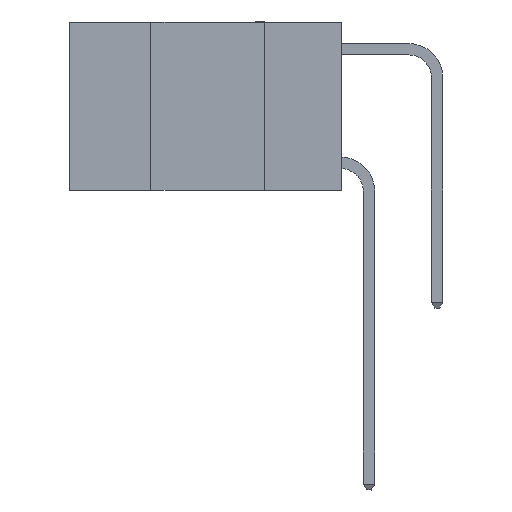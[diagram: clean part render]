
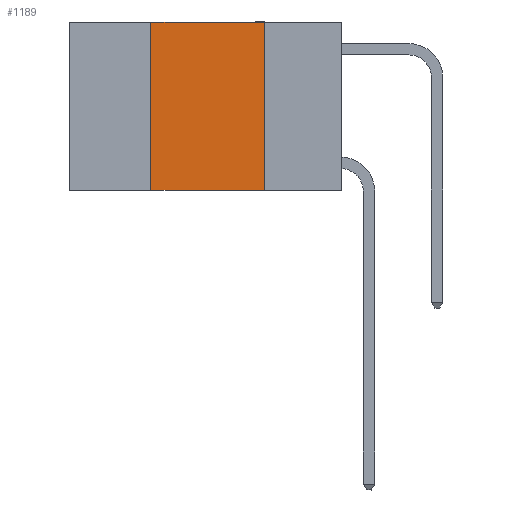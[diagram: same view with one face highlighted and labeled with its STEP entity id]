
A CAD part, left-side view. The second image highlights one B-rep face of the part: STEP entity #1189.
In plain terms, the highlighted planar face has unit normal (-1, 0, 0).
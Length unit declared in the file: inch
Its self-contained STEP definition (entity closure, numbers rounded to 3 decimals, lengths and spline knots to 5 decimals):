
#55 = EDGE_CURVE ( 'NONE', #11336, #14177, #9140, .T. ) ;
#119 = CARTESIAN_POINT ( 'NONE',  ( 0., 0.17, 0. ) ) ;
#1168 = CARTESIAN_POINT ( 'NONE',  ( 0., 0.42, -0.37 ) ) ;
#1189 = ADVANCED_FACE ( 'NONE', ( #21513 ), #1323, .F. ) ;
#1234 = DIRECTION ( 'NONE',  ( 1., 0., 0. ) ) ;
#1323 = PLANE ( 'NONE',  #14201 ) ;
#1516 = EDGE_CURVE ( 'NONE', #2004, #18646, #24204, .T. ) ;
#2004 = VERTEX_POINT ( 'NONE', #119 ) ;
#3366 = VECTOR ( 'NONE', #3903, 39.37008 ) ;
#3903 = DIRECTION ( 'NONE',  ( 0., 0., 1. ) ) ;
#5023 = DIRECTION ( 'NONE',  ( 0., 0., -1. ) ) ;
#6487 = CARTESIAN_POINT ( 'NONE',  ( 0., 0.6, 0. ) ) ;
#6698 = CARTESIAN_POINT ( 'NONE',  ( 0., 0.42, 0. ) ) ;
#7587 = VECTOR ( 'NONE', #21124, 39.37008 ) ;
#8258 = CARTESIAN_POINT ( 'NONE',  ( 0., 0.6, 0. ) ) ;
#9003 = ORIENTED_EDGE ( 'NONE', *, *, #16779, .F. ) ;
#9140 = LINE ( 'NONE', #18995, #3366 ) ;
#10365 = ORIENTED_EDGE ( 'NONE', *, *, #25208, .T. ) ;
#11336 = VERTEX_POINT ( 'NONE', #1168 ) ;
#14177 = VERTEX_POINT ( 'NONE', #6698 ) ;
#14201 = AXIS2_PLACEMENT_3D ( 'NONE', #6487, #1234, #22298 ) ;
#14974 = EDGE_LOOP ( 'NONE', ( #25488, #9003, #26829, #10365 ) ) ;
#15776 = CARTESIAN_POINT ( 'NONE',  ( 0., 0.17, 0. ) ) ;
#15861 = VECTOR ( 'NONE', #26058, 39.37008 ) ;
#16779 = EDGE_CURVE ( 'NONE', #14177, #2004, #19012, .T. ) ;
#18646 = VERTEX_POINT ( 'NONE', #22838 ) ;
#18995 = CARTESIAN_POINT ( 'NONE',  ( 0., 0.42, 0. ) ) ;
#19012 = LINE ( 'NONE', #8258, #7587 ) ;
#19569 = CARTESIAN_POINT ( 'NONE',  ( 0., 0.6, -0.37 ) ) ;
#21124 = DIRECTION ( 'NONE',  ( 0., -1., 0. ) ) ;
#21513 = FACE_OUTER_BOUND ( 'NONE', #14974, .T. ) ;
#22298 = DIRECTION ( 'NONE',  ( 0., 0., -1. ) ) ;
#22838 = CARTESIAN_POINT ( 'NONE',  ( 0., 0.17, -0.37 ) ) ;
#23535 = VECTOR ( 'NONE', #5023, 39.37008 ) ;
#24204 = LINE ( 'NONE', #15776, #23535 ) ;
#25208 = EDGE_CURVE ( 'NONE', #11336, #18646, #27295, .T. ) ;
#25488 = ORIENTED_EDGE ( 'NONE', *, *, #1516, .F. ) ;
#26058 = DIRECTION ( 'NONE',  ( 0., -1., 0. ) ) ;
#26829 = ORIENTED_EDGE ( 'NONE', *, *, #55, .F. ) ;
#27295 = LINE ( 'NONE', #19569, #15861 ) ;
